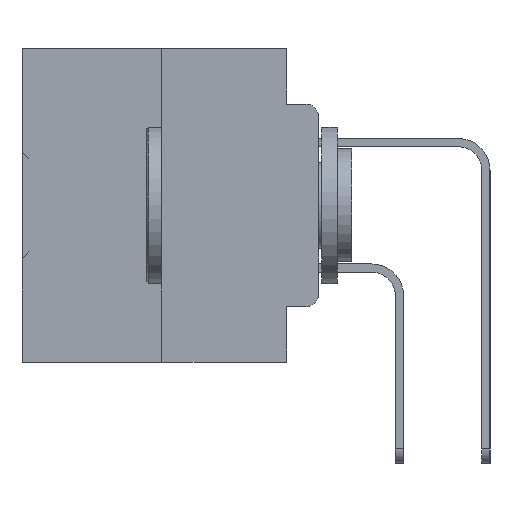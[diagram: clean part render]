
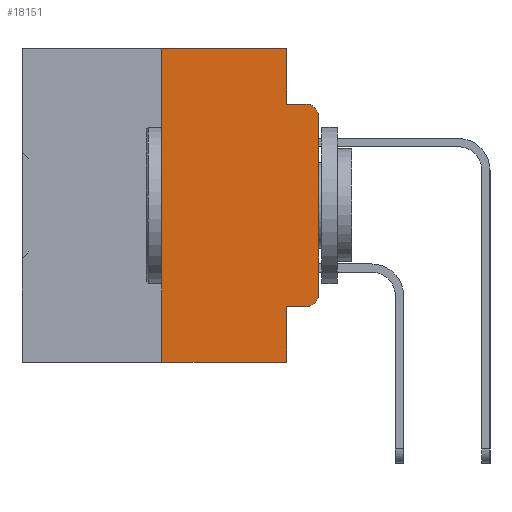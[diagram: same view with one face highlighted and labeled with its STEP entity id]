
A CAD part, left-side view. The second image highlights one B-rep face of the part: STEP entity #18151.
In plain terms, the highlighted planar face has unit normal (-1, 0, 0).
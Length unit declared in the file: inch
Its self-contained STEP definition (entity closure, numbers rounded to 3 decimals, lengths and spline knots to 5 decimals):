
#351 = LINE ( 'NONE', #32090, #19218 ) ;
#548 = DIRECTION ( 'NONE',  ( 0., 0., -1. ) ) ;
#751 = ORIENTED_EDGE ( 'NONE', *, *, #40811, .F. ) ;
#1064 = DIRECTION ( 'NONE',  ( 0., 0., -1. ) ) ;
#1580 = LINE ( 'NONE', #7837, #8040 ) ;
#2114 = DIRECTION ( 'NONE',  ( 0., 0., -1. ) ) ;
#2333 = LINE ( 'NONE', #38426, #18249 ) ;
#3149 = CARTESIAN_POINT ( 'NONE',  ( 0., 0.25, 0. ) ) ;
#3179 = EDGE_CURVE ( 'NONE', #14802, #38799, #351, .T. ) ;
#3251 = ORIENTED_EDGE ( 'NONE', *, *, #3179, .F. ) ;
#3437 = AXIS2_PLACEMENT_3D ( 'NONE', #38969, #20112, #1064 ) ;
#3647 = CARTESIAN_POINT ( 'NONE',  ( 0., 0., -0.1085 ) ) ;
#4872 = VERTEX_POINT ( 'NONE', #15765 ) ;
#5292 = EDGE_CURVE ( 'NONE', #37233, #38799, #30949, .T. ) ;
#5461 = CARTESIAN_POINT ( 'NONE',  ( 0., 0.051, -0.5 ) ) ;
#5806 = CARTESIAN_POINT ( 'NONE',  ( 0., 0.25, 0. ) ) ;
#6876 = EDGE_CURVE ( 'NONE', #4872, #32999, #15460, .T. ) ;
#7113 = EDGE_LOOP ( 'NONE', ( #26669, #19685, #3251, #751, #16111, #32852, #30380, #33784, #40169, #37656 ) ) ;
#7147 = VERTEX_POINT ( 'NONE', #5461 ) ;
#7419 = VERTEX_POINT ( 'NONE', #29075 ) ;
#7683 = CARTESIAN_POINT ( 'NONE',  ( 0., 0.051, 0. ) ) ;
#7837 = CARTESIAN_POINT ( 'NONE',  ( 0., 0.473, 0. ) ) ;
#8040 = VECTOR ( 'NONE', #20501, 39.37008 ) ;
#8563 = DIRECTION ( 'NONE',  ( 0., 0., 1. ) ) ;
#8882 = DIRECTION ( 'NONE',  ( 0., -1., 0. ) ) ;
#9026 = EDGE_CURVE ( 'NONE', #7419, #4872, #35166, .T. ) ;
#10449 = VECTOR ( 'NONE', #8563, 39.37008 ) ;
#10915 = DIRECTION ( 'NONE',  ( 0., 0., -1. ) ) ;
#10943 = CARTESIAN_POINT ( 'NONE',  ( 0., 0.051, -0.4115 ) ) ;
#13129 = DIRECTION ( 'NONE',  ( 0., -1., 0. ) ) ;
#14079 = VECTOR ( 'NONE', #10915, 39.37008 ) ;
#14247 = CARTESIAN_POINT ( 'NONE',  ( 0., 0.051, 0. ) ) ;
#14802 = VERTEX_POINT ( 'NONE', #27596 ) ;
#14817 = VERTEX_POINT ( 'NONE', #18164 ) ;
#15119 = VECTOR ( 'NONE', #31701, 39.37008 ) ;
#15191 = VERTEX_POINT ( 'NONE', #14247 ) ;
#15460 = CIRCLE ( 'NONE', #3437, 0.02 ) ;
#15765 = CARTESIAN_POINT ( 'NONE',  ( 0., 0.02, -0.4115 ) ) ;
#15943 = EDGE_CURVE ( 'NONE', #32999, #37233, #29299, .T. ) ;
#16111 = ORIENTED_EDGE ( 'NONE', *, *, #29260, .F. ) ;
#16851 = DIRECTION ( 'NONE',  ( 0., 0., -1. ) ) ;
#17534 = EDGE_CURVE ( 'NONE', #7419, #7147, #2333, .T. ) ;
#18010 = CARTESIAN_POINT ( 'NONE',  ( 0., 0., 0. ) ) ;
#18151 = ADVANCED_FACE ( 'NONE', ( #37973 ), #23170, .F. ) ;
#18164 = CARTESIAN_POINT ( 'NONE',  ( 0., 0.25, -0.5 ) ) ;
#18249 = VECTOR ( 'NONE', #548, 39.37008 ) ;
#18555 = VECTOR ( 'NONE', #8882, 39.37008 ) ;
#19218 = VECTOR ( 'NONE', #13129, 39.37008 ) ;
#19557 = LINE ( 'NONE', #40395, #18555 ) ;
#19685 = ORIENTED_EDGE ( 'NONE', *, *, #5292, .T. ) ;
#19688 = EDGE_CURVE ( 'NONE', #14817, #26219, #40338, .T. ) ;
#20112 = DIRECTION ( 'NONE',  ( -1., 0., 0. ) ) ;
#20501 = DIRECTION ( 'NONE',  ( 0., -1., 0. ) ) ;
#21176 = DIRECTION ( 'NONE',  ( -1., 0., 0. ) ) ;
#22446 = EDGE_CURVE ( 'NONE', #14817, #7147, #19557, .T. ) ;
#23170 = PLANE ( 'NONE',  #32389 ) ;
#23947 = CARTESIAN_POINT ( 'NONE',  ( 0., 0., -0.3915 ) ) ;
#24848 = VECTOR ( 'NONE', #30042, 39.37008 ) ;
#26219 = VERTEX_POINT ( 'NONE', #5806 ) ;
#26669 = ORIENTED_EDGE ( 'NONE', *, *, #15943, .T. ) ;
#27596 = CARTESIAN_POINT ( 'NONE',  ( 0., 0.051, -0.0885 ) ) ;
#27834 = CARTESIAN_POINT ( 'NONE',  ( 0., 0.02, -0.0885 ) ) ;
#29075 = CARTESIAN_POINT ( 'NONE',  ( 0., 0.051, -0.4115 ) ) ;
#29260 = EDGE_CURVE ( 'NONE', #26219, #15191, #1580, .T. ) ;
#29299 = LINE ( 'NONE', #18010, #10449 ) ;
#29481 = CARTESIAN_POINT ( 'NONE',  ( 0., 0.473, 0. ) ) ;
#30042 = DIRECTION ( 'NONE',  ( 0., -1., 0. ) ) ;
#30380 = ORIENTED_EDGE ( 'NONE', *, *, #22446, .T. ) ;
#30949 = CIRCLE ( 'NONE', #37842, 0.02 ) ;
#31701 = DIRECTION ( 'NONE',  ( 0., 0., 1. ) ) ;
#32090 = CARTESIAN_POINT ( 'NONE',  ( 0., 0.051, -0.0885 ) ) ;
#32389 = AXIS2_PLACEMENT_3D ( 'NONE', #29481, #35762, #16851 ) ;
#32852 = ORIENTED_EDGE ( 'NONE', *, *, #19688, .F. ) ;
#32999 = VERTEX_POINT ( 'NONE', #23947 ) ;
#33784 = ORIENTED_EDGE ( 'NONE', *, *, #17534, .F. ) ;
#35166 = LINE ( 'NONE', #10943, #24848 ) ;
#35762 = DIRECTION ( 'NONE',  ( 1., 0., 0. ) ) ;
#37233 = VERTEX_POINT ( 'NONE', #3647 ) ;
#37656 = ORIENTED_EDGE ( 'NONE', *, *, #6876, .T. ) ;
#37842 = AXIS2_PLACEMENT_3D ( 'NONE', #40021, #21176, #2114 ) ;
#37973 = FACE_OUTER_BOUND ( 'NONE', #7113, .T. ) ;
#38426 = CARTESIAN_POINT ( 'NONE',  ( 0., 0.051, 0. ) ) ;
#38799 = VERTEX_POINT ( 'NONE', #27834 ) ;
#38969 = CARTESIAN_POINT ( 'NONE',  ( 0., 0.02, -0.3915 ) ) ;
#39272 = LINE ( 'NONE', #7683, #14079 ) ;
#40021 = CARTESIAN_POINT ( 'NONE',  ( 0., 0.02, -0.1085 ) ) ;
#40169 = ORIENTED_EDGE ( 'NONE', *, *, #9026, .T. ) ;
#40338 = LINE ( 'NONE', #3149, #15119 ) ;
#40395 = CARTESIAN_POINT ( 'NONE',  ( 0., 0.473, -0.5 ) ) ;
#40811 = EDGE_CURVE ( 'NONE', #15191, #14802, #39272, .T. ) ;
